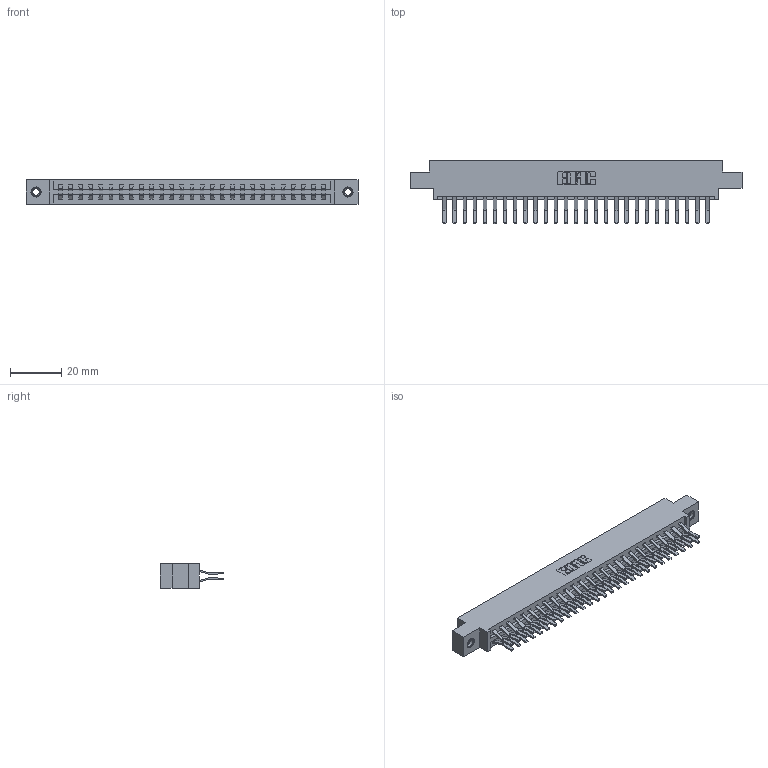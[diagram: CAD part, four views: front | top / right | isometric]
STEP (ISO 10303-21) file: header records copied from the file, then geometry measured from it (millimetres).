
FILE_DESCRIPTION (( 'STEP AP203' ), '1' );
FILE_NAME ('337-054-560-807.STEP', '2018-08-10T01:59:04', ( '' ), ( '' ), 'SwSTEP 2.0', 'SolidWorks 2016', '' );
FILE_SCHEMA (( 'CONFIG_CONTROL_DESIGN' ));
Length unit declared in the file: inch
Products named in the file (4): 337 Part_0.170 Offset - 0.156 Dia-TI; 345-292-001_560 Tail; 345-250-001_345-250-005-103; 337-054-560-807
Assembly tree (57 placements, depth 2):
  337-054-560-807
    337 Part_0.170 Offset - 0.156 Dia-TI
    345-292-001_560 Tail  x54
    345-250-001_345-250-005-103  x2
Bounding box: 130 x 24.78 x 9.4 mm (x, y, z)
Volume: 13723.4 mm3; surface area: 16536.8 mm2
Topology: 57 solids, 57 shells, 3202 faces, 9477 edges, 6238 vertices
Faces by surface type: plane 2158, cylinder 1028, cone 12, torus 4
Entity records: 24280 total; most frequent: CARTESIAN_POINT 4085, ORIENTED_EDGE 4014, DIRECTION 3537, EDGE_CURVE 2007, LINE 1855, VECTOR 1855, VERTEX_POINT 1332, AXIS2_PLACEMENT_3D 841
